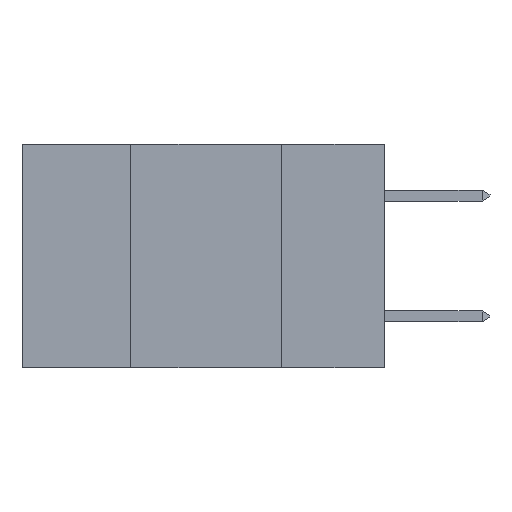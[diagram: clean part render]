
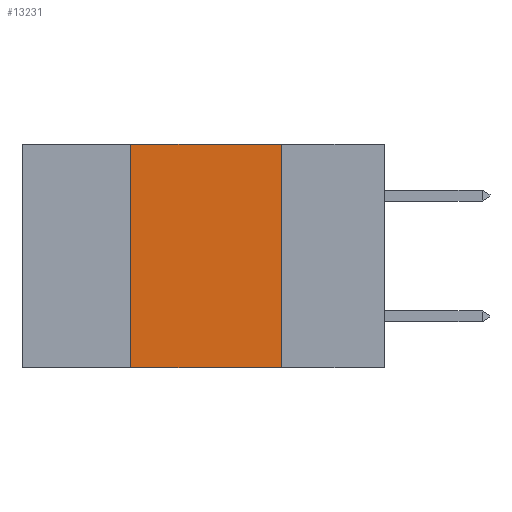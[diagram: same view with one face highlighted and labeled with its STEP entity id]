
A CAD part, left-side view. The second image highlights one B-rep face of the part: STEP entity #13231.
In plain terms, the highlighted planar face has unit normal (-1, 0, 0).
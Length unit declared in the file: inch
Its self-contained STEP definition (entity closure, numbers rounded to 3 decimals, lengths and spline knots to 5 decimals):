
#597 = DIRECTION ( 'NONE',  ( 0., -1., 0. ) ) ;
#2261 = AXIS2_PLACEMENT_3D ( 'NONE', #16869, #18812, #7275 ) ;
#2803 = ORIENTED_EDGE ( 'NONE', *, *, #17936, .F. ) ;
#3137 = CARTESIAN_POINT ( 'NONE',  ( 0., 0.17, 0. ) ) ;
#3419 = PLANE ( 'NONE',  #2261 ) ;
#3885 = LINE ( 'NONE', #22217, #14115 ) ;
#4331 = VERTEX_POINT ( 'NONE', #3137 ) ;
#5257 = VECTOR ( 'NONE', #597, 39.37008 ) ;
#5869 = LINE ( 'NONE', #23506, #5257 ) ;
#6402 = ORIENTED_EDGE ( 'NONE', *, *, #7674, .F. ) ;
#7275 = DIRECTION ( 'NONE',  ( 0., 0., -1. ) ) ;
#7674 = EDGE_CURVE ( 'NONE', #4331, #8188, #3885, .T. ) ;
#7846 = VECTOR ( 'NONE', #17040, 39.37008 ) ;
#8158 = FACE_OUTER_BOUND ( 'NONE', #13031, .T. ) ;
#8188 = VERTEX_POINT ( 'NONE', #10252 ) ;
#8451 = LINE ( 'NONE', #22746, #7846 ) ;
#9229 = DIRECTION ( 'NONE',  ( 0., -1., 0. ) ) ;
#10252 = CARTESIAN_POINT ( 'NONE',  ( 0., 0.17, -0.37 ) ) ;
#10779 = DIRECTION ( 'NONE',  ( 0., 0., -1. ) ) ;
#12175 = LINE ( 'NONE', #20708, #22341 ) ;
#12447 = CARTESIAN_POINT ( 'NONE',  ( 0., 0.42, -0.37 ) ) ;
#13031 = EDGE_LOOP ( 'NONE', ( #6402, #17250, #2803, #23738 ) ) ;
#13231 = ADVANCED_FACE ( 'NONE', ( #8158 ), #3419, .F. ) ;
#14115 = VECTOR ( 'NONE', #10779, 39.37008 ) ;
#14849 = EDGE_CURVE ( 'NONE', #18309, #4331, #5869, .T. ) ;
#16869 = CARTESIAN_POINT ( 'NONE',  ( 0., 0.6, 0. ) ) ;
#17040 = DIRECTION ( 'NONE',  ( 0., 0., 1. ) ) ;
#17250 = ORIENTED_EDGE ( 'NONE', *, *, #14849, .F. ) ;
#17936 = EDGE_CURVE ( 'NONE', #20277, #18309, #8451, .T. ) ;
#18309 = VERTEX_POINT ( 'NONE', #19945 ) ;
#18812 = DIRECTION ( 'NONE',  ( 1., 0., 0. ) ) ;
#19945 = CARTESIAN_POINT ( 'NONE',  ( 0., 0.42, 0. ) ) ;
#20277 = VERTEX_POINT ( 'NONE', #12447 ) ;
#20708 = CARTESIAN_POINT ( 'NONE',  ( 0., 0.6, -0.37 ) ) ;
#22217 = CARTESIAN_POINT ( 'NONE',  ( 0., 0.17, 0. ) ) ;
#22341 = VECTOR ( 'NONE', #9229, 39.37008 ) ;
#22746 = CARTESIAN_POINT ( 'NONE',  ( 0., 0.42, 0. ) ) ;
#23506 = CARTESIAN_POINT ( 'NONE',  ( 0., 0.6, 0. ) ) ;
#23738 = ORIENTED_EDGE ( 'NONE', *, *, #24382, .T. ) ;
#24382 = EDGE_CURVE ( 'NONE', #20277, #8188, #12175, .T. ) ;
